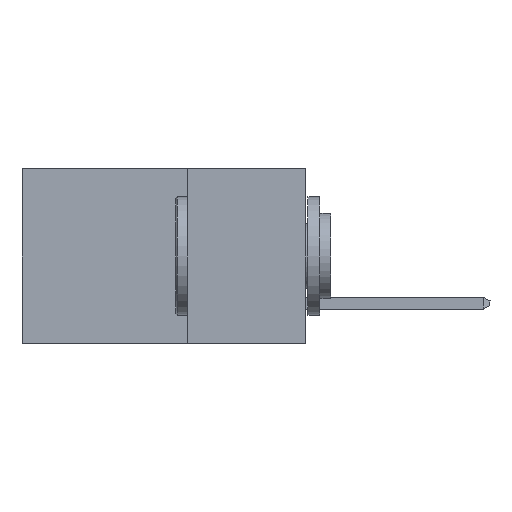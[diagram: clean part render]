
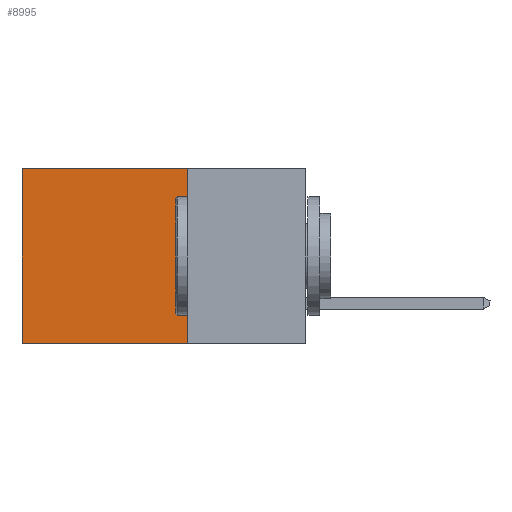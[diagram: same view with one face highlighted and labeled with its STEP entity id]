
A CAD part, left-side view. The second image highlights one B-rep face of the part: STEP entity #8995.
In plain terms, the highlighted planar face has unit normal (-1, 0, 0).
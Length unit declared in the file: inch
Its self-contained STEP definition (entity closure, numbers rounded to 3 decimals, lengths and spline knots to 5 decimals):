
#870 = ORIENTED_EDGE ( 'NONE', *, *, #2015, .F. ) ;
#1210 = DIRECTION ( 'NONE',  ( 0., 0., -1. ) ) ;
#1316 = CARTESIAN_POINT ( 'NONE',  ( 0.2615, 0.25, 0. ) ) ;
#1424 = LINE ( 'NONE', #4359, #3100 ) ;
#1618 = VERTEX_POINT ( 'NONE', #15618 ) ;
#2015 = EDGE_CURVE ( 'NONE', #1618, #14619, #1424, .T. ) ;
#3017 = FACE_OUTER_BOUND ( 'NONE', #18880, .T. ) ;
#3100 = VECTOR ( 'NONE', #10707, 39.37008 ) ;
#3774 = VERTEX_POINT ( 'NONE', #18968 ) ;
#3827 = LINE ( 'NONE', #5613, #9850 ) ;
#4359 = CARTESIAN_POINT ( 'NONE',  ( 0.2615, 0.25, -0.37 ) ) ;
#4799 = PLANE ( 'NONE',  #20432 ) ;
#4861 = ORIENTED_EDGE ( 'NONE', *, *, #16511, .T. ) ;
#5613 = CARTESIAN_POINT ( 'NONE',  ( 0.2615, 0.6, -0.37 ) ) ;
#6880 = CARTESIAN_POINT ( 'NONE',  ( 0.2615, 0.6, -0.37 ) ) ;
#7483 = VECTOR ( 'NONE', #15485, 39.37008 ) ;
#8123 = DIRECTION ( 'NONE',  ( 0., 0., -1. ) ) ;
#8995 = ADVANCED_FACE ( 'NONE', ( #3017 ), #4799, .F. ) ;
#9582 = DIRECTION ( 'NONE',  ( 1., 0., 0. ) ) ;
#9850 = VECTOR ( 'NONE', #10189, 39.37008 ) ;
#10189 = DIRECTION ( 'NONE',  ( 0., 0., -1. ) ) ;
#10707 = DIRECTION ( 'NONE',  ( 0., 1., 0. ) ) ;
#11676 = CARTESIAN_POINT ( 'NONE',  ( 0.2615, 0.25, 0. ) ) ;
#13249 = VECTOR ( 'NONE', #1210, 39.37008 ) ;
#14619 = VERTEX_POINT ( 'NONE', #6880 ) ;
#14901 = EDGE_CURVE ( 'NONE', #17717, #1618, #15078, .T. ) ;
#15078 = LINE ( 'NONE', #15478, #13249 ) ;
#15478 = CARTESIAN_POINT ( 'NONE',  ( 0.2615, 0.25, -0.37 ) ) ;
#15485 = DIRECTION ( 'NONE',  ( 0., 1., 0. ) ) ;
#15618 = CARTESIAN_POINT ( 'NONE',  ( 0.2615, 0.25, -0.37 ) ) ;
#16511 = EDGE_CURVE ( 'NONE', #17717, #3774, #17149, .T. ) ;
#17149 = LINE ( 'NONE', #1316, #7483 ) ;
#17477 = CARTESIAN_POINT ( 'NONE',  ( 0.2615, 0.25, -0.37 ) ) ;
#17717 = VERTEX_POINT ( 'NONE', #11676 ) ;
#17835 = ORIENTED_EDGE ( 'NONE', *, *, #18067, .T. ) ;
#18067 = EDGE_CURVE ( 'NONE', #3774, #14619, #3827, .T. ) ;
#18395 = ORIENTED_EDGE ( 'NONE', *, *, #14901, .F. ) ;
#18880 = EDGE_LOOP ( 'NONE', ( #17835, #870, #18395, #4861 ) ) ;
#18968 = CARTESIAN_POINT ( 'NONE',  ( 0.2615, 0.6, 0. ) ) ;
#20432 = AXIS2_PLACEMENT_3D ( 'NONE', #17477, #9582, #8123 ) ;
